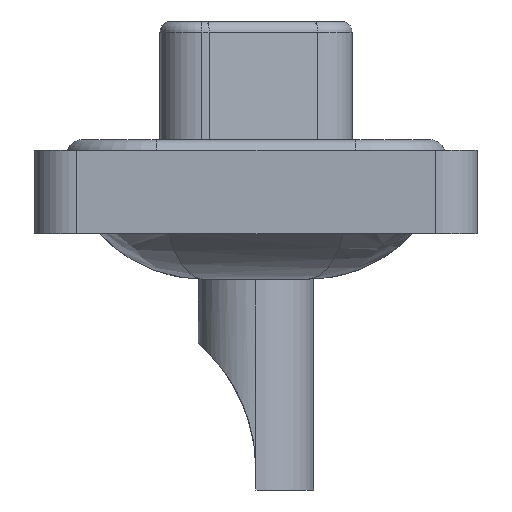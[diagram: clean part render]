
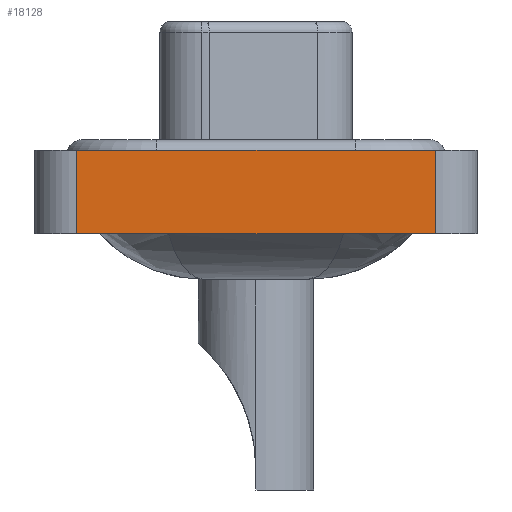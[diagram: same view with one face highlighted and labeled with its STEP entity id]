
A CAD part, left-side view. The second image highlights one B-rep face of the part: STEP entity #18128.
In plain terms, the highlighted planar face has unit normal (-1, 0, 0).
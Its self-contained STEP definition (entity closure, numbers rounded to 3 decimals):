
#1173 = EDGE_LOOP ( 'NONE', ( #3895, #16561, #6309, #9657 ) ) ;
#1899 = DIRECTION ( 'NONE',  ( 0., 0., 1. ) ) ;
#2541 = LINE ( 'NONE', #20564, #14594 ) ;
#2851 = VERTEX_POINT ( 'NONE', #22416 ) ;
#2960 = DIRECTION ( 'NONE',  ( 0., 0., 1. ) ) ;
#3895 = ORIENTED_EDGE ( 'NONE', *, *, #12489, .T. ) ;
#4630 = VECTOR ( 'NONE', #2960, 1000. ) ;
#5173 = VECTOR ( 'NONE', #16165, 1000. ) ;
#5578 = PLANE ( 'NONE',  #14553 ) ;
#5811 = DIRECTION ( 'NONE',  ( -1., 0., 0. ) ) ;
#6266 = VERTEX_POINT ( 'NONE', #21487 ) ;
#6309 = ORIENTED_EDGE ( 'NONE', *, *, #15390, .F. ) ;
#6888 = CARTESIAN_POINT ( 'NONE',  ( -7.35, -8.55, -3.6 ) ) ;
#7816 = EDGE_CURVE ( 'NONE', #6266, #13579, #2541, .T. ) ;
#9657 = ORIENTED_EDGE ( 'NONE', *, *, #7816, .T. ) ;
#9740 = DIRECTION ( 'NONE',  ( 0., -1., 0. ) ) ;
#11086 = LINE ( 'NONE', #16524, #22086 ) ;
#12426 = EDGE_CURVE ( 'NONE', #12471, #2851, #20897, .T. ) ;
#12471 = VERTEX_POINT ( 'NONE', #14992 ) ;
#12489 = EDGE_CURVE ( 'NONE', #13579, #2851, #11086, .T. ) ;
#13121 = FACE_OUTER_BOUND ( 'NONE', #1173, .T. ) ;
#13579 = VERTEX_POINT ( 'NONE', #6888 ) ;
#14553 = AXIS2_PLACEMENT_3D ( 'NONE', #18426, #5811, #16312 ) ;
#14594 = VECTOR ( 'NONE', #9740, 1000. ) ;
#14992 = CARTESIAN_POINT ( 'NONE',  ( -7.35, 8.55, 0.4 ) ) ;
#15390 = EDGE_CURVE ( 'NONE', #6266, #12471, #16863, .T. ) ;
#16165 = DIRECTION ( 'NONE',  ( 0., -1., 0. ) ) ;
#16312 = DIRECTION ( 'NONE',  ( 0., 0., 1. ) ) ;
#16524 = CARTESIAN_POINT ( 'NONE',  ( -7.35, -8.55, -3.6 ) ) ;
#16561 = ORIENTED_EDGE ( 'NONE', *, *, #12426, .F. ) ;
#16863 = LINE ( 'NONE', #20848, #4630 ) ;
#18128 = ADVANCED_FACE ( 'NONE', ( #13121 ), #5578, .T. ) ;
#18426 = CARTESIAN_POINT ( 'NONE',  ( -7.35, -8.55, -3.6 ) ) ;
#19674 = CARTESIAN_POINT ( 'NONE',  ( -7.35, -8.55, 0.4 ) ) ;
#20564 = CARTESIAN_POINT ( 'NONE',  ( -7.35, -8.55, -3.6 ) ) ;
#20848 = CARTESIAN_POINT ( 'NONE',  ( -7.35, 8.55, -3.6 ) ) ;
#20897 = LINE ( 'NONE', #19674, #5173 ) ;
#21487 = CARTESIAN_POINT ( 'NONE',  ( -7.35, 8.55, -3.6 ) ) ;
#22086 = VECTOR ( 'NONE', #1899, 1000. ) ;
#22416 = CARTESIAN_POINT ( 'NONE',  ( -7.35, -8.55, 0.4 ) ) ;
